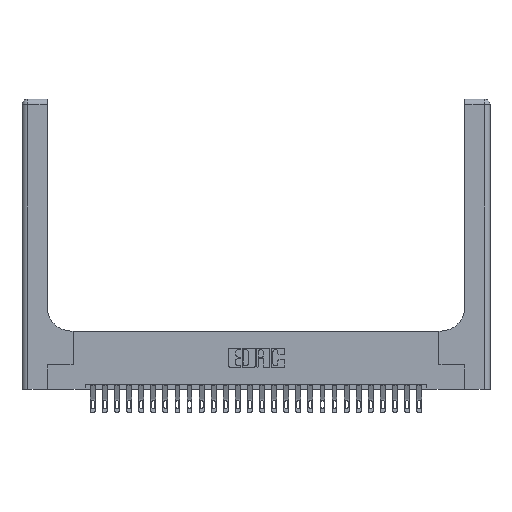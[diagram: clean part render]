
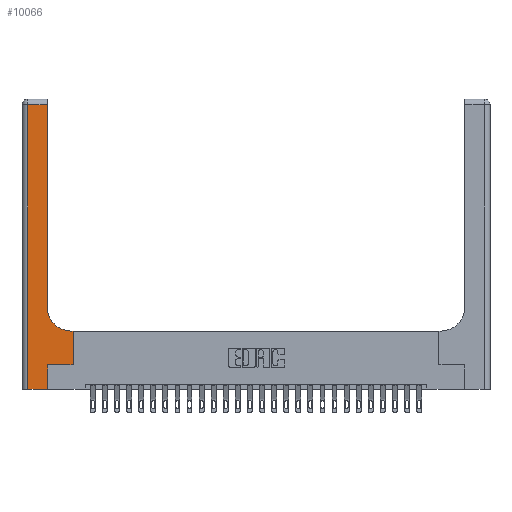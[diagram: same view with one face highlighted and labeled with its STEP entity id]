
A CAD part, top view. The second image highlights one B-rep face of the part: STEP entity #10066.
In plain terms, the highlighted planar face has unit normal (0, 0, 1).
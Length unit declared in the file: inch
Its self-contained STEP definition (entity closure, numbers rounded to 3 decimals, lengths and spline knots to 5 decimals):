
#278 = EDGE_CURVE ( 'NONE', #25282, #3573, #10599, .T. ) ;
#336 = FACE_OUTER_BOUND ( 'NONE', #9547, .T. ) ;
#1359 = ORIENTED_EDGE ( 'NONE', *, *, #1619, .T. ) ;
#1360 = CARTESIAN_POINT ( 'NONE',  ( 0.26, 2.94, 0.37 ) ) ;
#1516 = VECTOR ( 'NONE', #7562, 39.37008 ) ;
#1619 = EDGE_CURVE ( 'NONE', #22002, #16945, #5214, .T. ) ;
#1793 = LINE ( 'NONE', #6556, #25044 ) ;
#2158 = VECTOR ( 'NONE', #14973, 39.37008 ) ;
#2523 = EDGE_CURVE ( 'NONE', #3573, #22002, #17653, .T. ) ;
#3020 = CARTESIAN_POINT ( 'NONE',  ( 0.06, 0., 0.37 ) ) ;
#3243 = CARTESIAN_POINT ( 'NONE',  ( 0., 0., 0.37 ) ) ;
#3388 = ORIENTED_EDGE ( 'NONE', *, *, #14075, .T. ) ;
#3507 = CARTESIAN_POINT ( 'NONE',  ( 0., 3., 0.37 ) ) ;
#3573 = VERTEX_POINT ( 'NONE', #7193 ) ;
#3964 = CARTESIAN_POINT ( 'NONE',  ( 0.26, 3., 0.37 ) ) ;
#3997 = VECTOR ( 'NONE', #18853, 39.37008 ) ;
#4844 = DIRECTION ( 'NONE',  ( 0., 1., 0. ) ) ;
#4915 = EDGE_CURVE ( 'NONE', #25292, #5937, #17992, .T. ) ;
#4958 = CARTESIAN_POINT ( 'NONE',  ( 0.528, 0.6, 0.37 ) ) ;
#5214 = LINE ( 'NONE', #20910, #3997 ) ;
#5327 = ORIENTED_EDGE ( 'NONE', *, *, #278, .T. ) ;
#5937 = VERTEX_POINT ( 'NONE', #3020 ) ;
#6474 = DIRECTION ( 'NONE',  ( 0., 1., 0. ) ) ;
#6556 = CARTESIAN_POINT ( 'NONE',  ( 0.265, 0., 0.37 ) ) ;
#6956 = CARTESIAN_POINT ( 'NONE',  ( 0.51, 0.85, 0.37 ) ) ;
#7193 = CARTESIAN_POINT ( 'NONE',  ( 0.528, 0.25, 0.37 ) ) ;
#7327 = VECTOR ( 'NONE', #11132, 39.37008 ) ;
#7562 = DIRECTION ( 'NONE',  ( 0., -1., 0. ) ) ;
#7787 = VECTOR ( 'NONE', #10082, 39.37008 ) ;
#8892 = ORIENTED_EDGE ( 'NONE', *, *, #4915, .T. ) ;
#9547 = EDGE_LOOP ( 'NONE', ( #10338, #3388, #8892, #14334, #15262, #5327, #18094, #1359, #18511 ) ) ;
#9578 = CARTESIAN_POINT ( 'NONE',  ( 0.265, 0., 0.37 ) ) ;
#9621 = CARTESIAN_POINT ( 'NONE',  ( 0.51, 0.6, 0.37 ) ) ;
#10066 = ADVANCED_FACE ( 'NONE', ( #336 ), #11613, .F. ) ;
#10082 = DIRECTION ( 'NONE',  ( 1., 0., 0. ) ) ;
#10338 = ORIENTED_EDGE ( 'NONE', *, *, #20662, .T. ) ;
#10433 = CARTESIAN_POINT ( 'NONE',  ( 0.528, 0.25, 0.37 ) ) ;
#10599 = LINE ( 'NONE', #23755, #7787 ) ;
#11132 = DIRECTION ( 'NONE',  ( -1., 0., 0. ) ) ;
#11613 = PLANE ( 'NONE',  #23654 ) ;
#11772 = LINE ( 'NONE', #3243, #2158 ) ;
#12202 = VERTEX_POINT ( 'NONE', #9578 ) ;
#12675 = AXIS2_PLACEMENT_3D ( 'NONE', #6956, #17073, #17165 ) ;
#12845 = VECTOR ( 'NONE', #23495, 39.37008 ) ;
#12938 = EDGE_CURVE ( 'NONE', #5937, #12202, #11772, .T. ) ;
#12962 = EDGE_CURVE ( 'NONE', #16945, #20285, #16097, .T. ) ;
#13837 = EDGE_CURVE ( 'NONE', #12202, #25282, #1793, .T. ) ;
#14075 = EDGE_CURVE ( 'NONE', #15633, #25292, #21014, .T. ) ;
#14334 = ORIENTED_EDGE ( 'NONE', *, *, #12938, .T. ) ;
#14973 = DIRECTION ( 'NONE',  ( 1., 0., 0. ) ) ;
#15262 = ORIENTED_EDGE ( 'NONE', *, *, #13837, .T. ) ;
#15633 = VERTEX_POINT ( 'NONE', #1360 ) ;
#16097 = CIRCLE ( 'NONE', #12675, 0.25 ) ;
#16945 = VERTEX_POINT ( 'NONE', #9621 ) ;
#17073 = DIRECTION ( 'NONE',  ( 0., 0., -1. ) ) ;
#17165 = DIRECTION ( 'NONE',  ( 1., 0., 0. ) ) ;
#17653 = LINE ( 'NONE', #10433, #18903 ) ;
#17992 = LINE ( 'NONE', #23276, #1516 ) ;
#18094 = ORIENTED_EDGE ( 'NONE', *, *, #2523, .T. ) ;
#18356 = CARTESIAN_POINT ( 'NONE',  ( 0.06, 2.94, 0.37 ) ) ;
#18511 = ORIENTED_EDGE ( 'NONE', *, *, #12962, .T. ) ;
#18853 = DIRECTION ( 'NONE',  ( -1., 0., 0. ) ) ;
#18903 = VECTOR ( 'NONE', #4844, 39.37008 ) ;
#18963 = CARTESIAN_POINT ( 'NONE',  ( 0., 2.94, 0.37 ) ) ;
#20285 = VERTEX_POINT ( 'NONE', #21927 ) ;
#20662 = EDGE_CURVE ( 'NONE', #20285, #15633, #25542, .T. ) ;
#20910 = CARTESIAN_POINT ( 'NONE',  ( 0.26, 0.6, 0.37 ) ) ;
#21014 = LINE ( 'NONE', #18963, #7327 ) ;
#21927 = CARTESIAN_POINT ( 'NONE',  ( 0.26, 0.85, 0.37 ) ) ;
#22002 = VERTEX_POINT ( 'NONE', #4958 ) ;
#23276 = CARTESIAN_POINT ( 'NONE',  ( 0.06, 3., 0.37 ) ) ;
#23495 = DIRECTION ( 'NONE',  ( 0., 1., 0. ) ) ;
#23554 = DIRECTION ( 'NONE',  ( -1., 0., 0. ) ) ;
#23654 = AXIS2_PLACEMENT_3D ( 'NONE', #3507, #25472, #23554 ) ;
#23755 = CARTESIAN_POINT ( 'NONE',  ( 0.265, 0.25, 0.37 ) ) ;
#24050 = CARTESIAN_POINT ( 'NONE',  ( 0.265, 0.25, 0.37 ) ) ;
#25044 = VECTOR ( 'NONE', #6474, 39.37008 ) ;
#25282 = VERTEX_POINT ( 'NONE', #24050 ) ;
#25292 = VERTEX_POINT ( 'NONE', #18356 ) ;
#25472 = DIRECTION ( 'NONE',  ( 0., 0., -1. ) ) ;
#25542 = LINE ( 'NONE', #3964, #12845 ) ;
